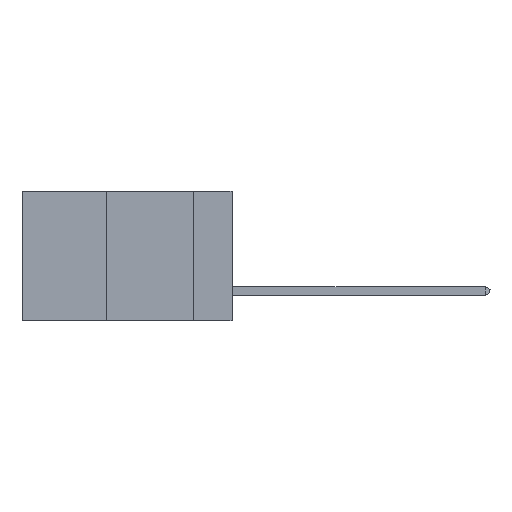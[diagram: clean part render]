
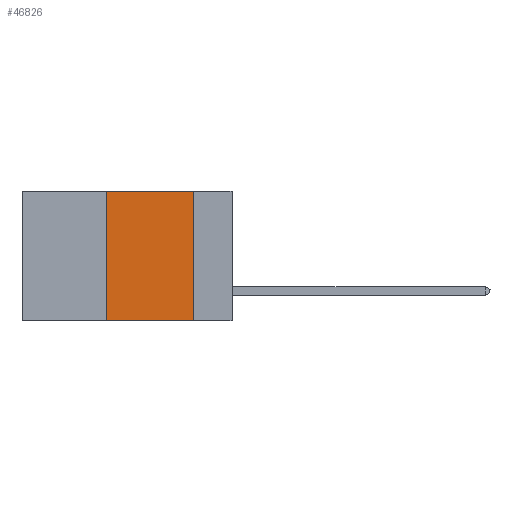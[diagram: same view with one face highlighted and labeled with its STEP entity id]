
A CAD part, left-side view. The second image highlights one B-rep face of the part: STEP entity #46826.
In plain terms, the highlighted planar face has unit normal (-1, 0, 0).
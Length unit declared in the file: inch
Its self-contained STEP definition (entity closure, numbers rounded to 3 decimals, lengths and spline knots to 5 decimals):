
#212 = DIRECTION ( 'NONE',  ( 0., -1., 0. ) ) ;
#4520 = ORIENTED_EDGE ( 'NONE', *, *, #34700, .T. ) ;
#8195 = VECTOR ( 'NONE', #45240, 39.37008 ) ;
#8788 = CARTESIAN_POINT ( 'NONE',  ( 0., 0.11, -0.37 ) ) ;
#8874 = LINE ( 'NONE', #23832, #15413 ) ;
#14442 = CARTESIAN_POINT ( 'NONE',  ( 0., 0.11, 0. ) ) ;
#15413 = VECTOR ( 'NONE', #44778, 39.37008 ) ;
#17511 = VECTOR ( 'NONE', #212, 39.37008 ) ;
#18890 = CARTESIAN_POINT ( 'NONE',  ( 0., 0.36, 0. ) ) ;
#19032 = DIRECTION ( 'NONE',  ( 0., 0., -1. ) ) ;
#19080 = ORIENTED_EDGE ( 'NONE', *, *, #39150, .F. ) ;
#19092 = DIRECTION ( 'NONE',  ( 1., 0., 0. ) ) ;
#19807 = EDGE_CURVE ( 'NONE', #32737, #45275, #8874, .T. ) ;
#21909 = VERTEX_POINT ( 'NONE', #8788 ) ;
#22179 = ORIENTED_EDGE ( 'NONE', *, *, #40598, .F. ) ;
#22873 = DIRECTION ( 'NONE',  ( 0., 0., -1. ) ) ;
#22876 = CARTESIAN_POINT ( 'NONE',  ( 0., 0.6, -0.37 ) ) ;
#23192 = AXIS2_PLACEMENT_3D ( 'NONE', #37815, #19092, #22873 ) ;
#23832 = CARTESIAN_POINT ( 'NONE',  ( 0., 0.6, 0. ) ) ;
#24085 = CARTESIAN_POINT ( 'NONE',  ( 0., 0.11, 0. ) ) ;
#28268 = LINE ( 'NONE', #18890, #8195 ) ;
#28396 = CARTESIAN_POINT ( 'NONE',  ( 0., 0.36, 0. ) ) ;
#30718 = PLANE ( 'NONE',  #23192 ) ;
#31318 = CARTESIAN_POINT ( 'NONE',  ( 0., 0.36, -0.37 ) ) ;
#32737 = VERTEX_POINT ( 'NONE', #28396 ) ;
#32842 = EDGE_LOOP ( 'NONE', ( #22179, #46368, #19080, #4520 ) ) ;
#33531 = LINE ( 'NONE', #14442, #41236 ) ;
#34700 = EDGE_CURVE ( 'NONE', #36268, #21909, #41151, .T. ) ;
#36268 = VERTEX_POINT ( 'NONE', #31318 ) ;
#37815 = CARTESIAN_POINT ( 'NONE',  ( 0., 0.6, 0. ) ) ;
#39150 = EDGE_CURVE ( 'NONE', #36268, #32737, #28268, .T. ) ;
#40598 = EDGE_CURVE ( 'NONE', #45275, #21909, #33531, .T. ) ;
#41151 = LINE ( 'NONE', #22876, #17511 ) ;
#41236 = VECTOR ( 'NONE', #19032, 39.37008 ) ;
#44778 = DIRECTION ( 'NONE',  ( 0., -1., 0. ) ) ;
#45067 = FACE_OUTER_BOUND ( 'NONE', #32842, .T. ) ;
#45240 = DIRECTION ( 'NONE',  ( 0., 0., 1. ) ) ;
#45275 = VERTEX_POINT ( 'NONE', #24085 ) ;
#46368 = ORIENTED_EDGE ( 'NONE', *, *, #19807, .F. ) ;
#46826 = ADVANCED_FACE ( 'NONE', ( #45067 ), #30718, .F. ) ;
